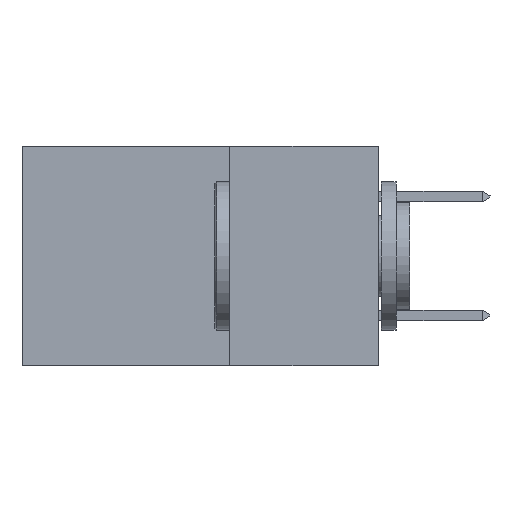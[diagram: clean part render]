
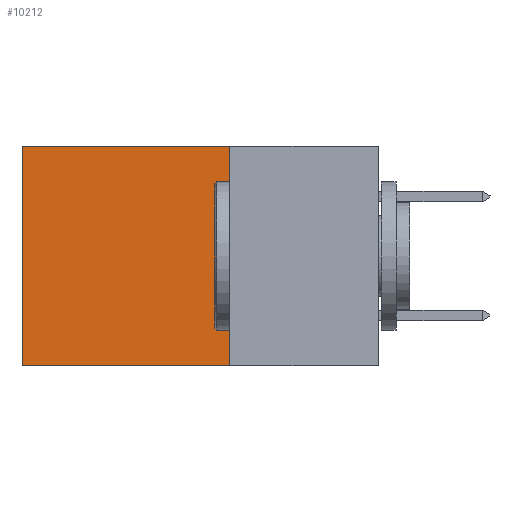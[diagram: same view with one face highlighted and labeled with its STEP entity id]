
A CAD part, left-side view. The second image highlights one B-rep face of the part: STEP entity #10212.
In plain terms, the highlighted planar face has unit normal (-1, 0, 0).
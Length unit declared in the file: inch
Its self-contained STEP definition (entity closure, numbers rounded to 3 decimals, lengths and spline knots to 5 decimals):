
#145 = ORIENTED_EDGE ( 'NONE', *, *, #4994, .T. ) ;
#284 = EDGE_CURVE ( 'NONE', #23576, #3853, #17677, .T. ) ;
#628 = DIRECTION ( 'NONE',  ( 0., 0., -1. ) ) ;
#881 = CARTESIAN_POINT ( 'NONE',  ( 0.2615, 0.25, 0. ) ) ;
#2449 = LINE ( 'NONE', #19241, #16021 ) ;
#2748 = CARTESIAN_POINT ( 'NONE',  ( 0.2615, 0.25, 0. ) ) ;
#3853 = VERTEX_POINT ( 'NONE', #9430 ) ;
#4552 = CARTESIAN_POINT ( 'NONE',  ( 0.2615, 0.25, -0.37 ) ) ;
#4994 = EDGE_CURVE ( 'NONE', #3853, #12971, #21720, .T. ) ;
#5514 = EDGE_CURVE ( 'NONE', #23576, #23344, #8816, .T. ) ;
#6566 = ORIENTED_EDGE ( 'NONE', *, *, #284, .T. ) ;
#7973 = CARTESIAN_POINT ( 'NONE',  ( 0.2615, 0.6, -0.37 ) ) ;
#8068 = AXIS2_PLACEMENT_3D ( 'NONE', #4552, #8226, #628 ) ;
#8226 = DIRECTION ( 'NONE',  ( 1., 0., 0. ) ) ;
#8246 = DIRECTION ( 'NONE',  ( 0., 1., 0. ) ) ;
#8472 = VECTOR ( 'NONE', #22462, 39.37008 ) ;
#8816 = LINE ( 'NONE', #16638, #16351 ) ;
#9430 = CARTESIAN_POINT ( 'NONE',  ( 0.2615, 0.6, 0. ) ) ;
#10212 = ADVANCED_FACE ( 'NONE', ( #22714 ), #20984, .F. ) ;
#10759 = DIRECTION ( 'NONE',  ( 0., 0., -1. ) ) ;
#12137 = ORIENTED_EDGE ( 'NONE', *, *, #5514, .F. ) ;
#12971 = VERTEX_POINT ( 'NONE', #7973 ) ;
#16021 = VECTOR ( 'NONE', #23057, 39.37008 ) ;
#16351 = VECTOR ( 'NONE', #10759, 39.37008 ) ;
#16638 = CARTESIAN_POINT ( 'NONE',  ( 0.2615, 0.25, -0.37 ) ) ;
#17677 = LINE ( 'NONE', #881, #18925 ) ;
#18590 = EDGE_LOOP ( 'NONE', ( #145, #20761, #12137, #6566 ) ) ;
#18824 = EDGE_CURVE ( 'NONE', #23344, #12971, #2449, .T. ) ;
#18925 = VECTOR ( 'NONE', #8246, 39.37008 ) ;
#19241 = CARTESIAN_POINT ( 'NONE',  ( 0.2615, 0.25, -0.37 ) ) ;
#19870 = CARTESIAN_POINT ( 'NONE',  ( 0.2615, 0.6, -0.37 ) ) ;
#20761 = ORIENTED_EDGE ( 'NONE', *, *, #18824, .F. ) ;
#20984 = PLANE ( 'NONE',  #8068 ) ;
#21720 = LINE ( 'NONE', #19870, #8472 ) ;
#22462 = DIRECTION ( 'NONE',  ( 0., 0., -1. ) ) ;
#22714 = FACE_OUTER_BOUND ( 'NONE', #18590, .T. ) ;
#23057 = DIRECTION ( 'NONE',  ( 0., 1., 0. ) ) ;
#23344 = VERTEX_POINT ( 'NONE', #24131 ) ;
#23576 = VERTEX_POINT ( 'NONE', #2748 ) ;
#24131 = CARTESIAN_POINT ( 'NONE',  ( 0.2615, 0.25, -0.37 ) ) ;
